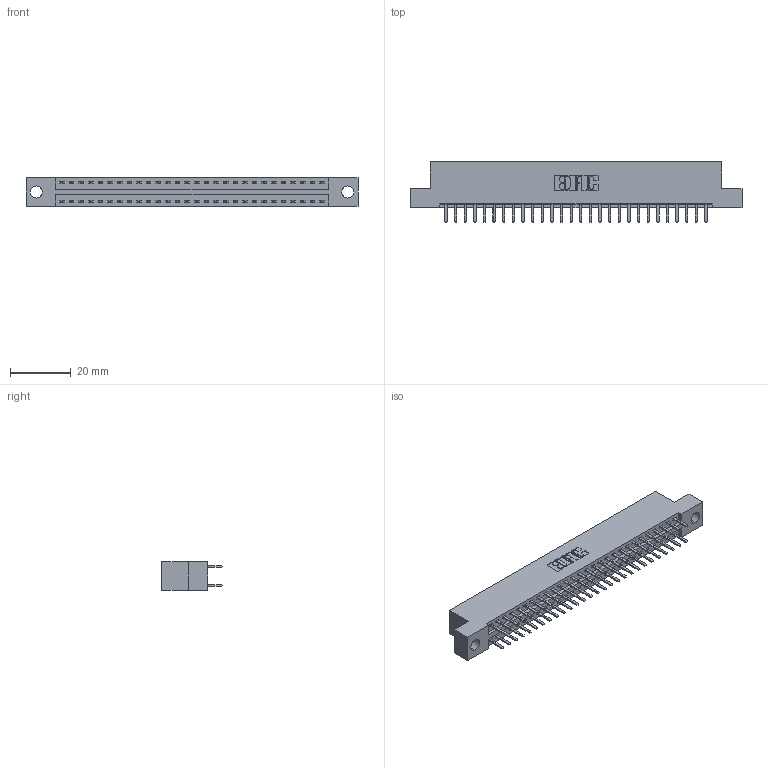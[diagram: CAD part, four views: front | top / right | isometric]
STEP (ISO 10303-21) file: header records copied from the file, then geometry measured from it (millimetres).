
FILE_DESCRIPTION (( 'STEP AP203' ), '1' );
FILE_NAME ('346-056-520-204.STEP', '2022-05-21T04:59:59', ( '' ), ( '' ), 'SwSTEP 2.0', 'SolidWorks 2020', '' );
FILE_SCHEMA (( 'CONFIG_CONTROL_DESIGN' ));
Length unit declared in the file: inch
Products named in the file (3): 346-056-520-204; 346 Part_Flush Mounting Lugs - 0.156 Dia-TH; 345-292-001_345-293-120
Assembly tree (57 placements, depth 2):
  346-056-520-204
    346 Part_Flush Mounting Lugs - 0.156 Dia-TH
    345-292-001_345-293-120  x56
Bounding box: 109.47 x 20.02 x 9.4 mm (x, y, z)
Volume: 10435.8 mm3; surface area: 13914.8 mm2
Topology: 57 solids, 57 shells, 3272 faces, 9493 edges, 6178 vertices
Faces by surface type: plane 2162, cylinder 1110
Entity records: 20691 total; most frequent: CARTESIAN_POINT 3446, ORIENTED_EDGE 3366, DIRECTION 3075, EDGE_CURVE 1683, LINE 1435, VECTOR 1435, VERTEX_POINT 1118, AXIS2_PLACEMENT_3D 820
